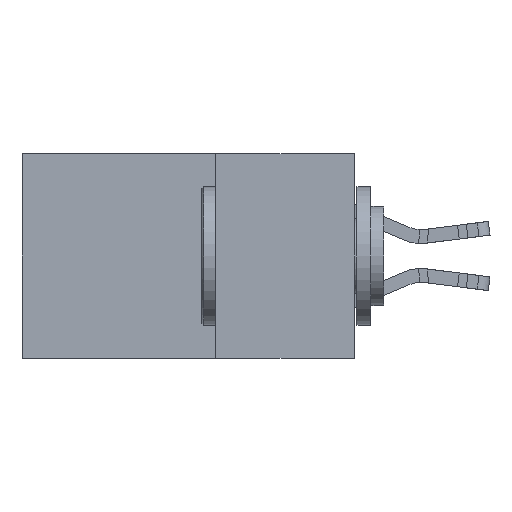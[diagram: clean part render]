
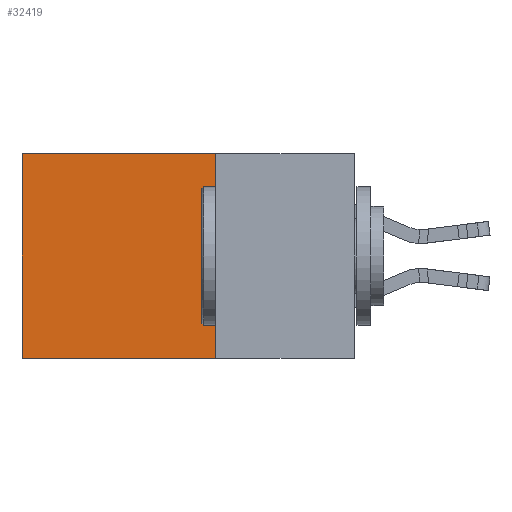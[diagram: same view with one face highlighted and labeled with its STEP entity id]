
A CAD part, left-side view. The second image highlights one B-rep face of the part: STEP entity #32419.
In plain terms, the highlighted planar face has unit normal (-1, 0, 0).
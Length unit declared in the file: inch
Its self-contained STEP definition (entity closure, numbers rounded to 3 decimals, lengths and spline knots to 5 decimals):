
#545 = EDGE_CURVE ( 'NONE', #3159, #31129, #23903, .T. ) ;
#954 = AXIS2_PLACEMENT_3D ( 'NONE', #7554, #33382, #17933 ) ;
#1598 = VECTOR ( 'NONE', #5966, 39.37008 ) ;
#2440 = DIRECTION ( 'NONE',  ( 0., 0., -1. ) ) ;
#2463 = CARTESIAN_POINT ( 'NONE',  ( 0.298, 0.25, -0.37 ) ) ;
#3159 = VERTEX_POINT ( 'NONE', #21073 ) ;
#3337 = DIRECTION ( 'NONE',  ( 0., 0., -1. ) ) ;
#4181 = ORIENTED_EDGE ( 'NONE', *, *, #545, .T. ) ;
#4234 = CARTESIAN_POINT ( 'NONE',  ( 0.298, 0.6, -0.37 ) ) ;
#5095 = CARTESIAN_POINT ( 'NONE',  ( 0.298, 0.25, 0. ) ) ;
#5665 = VECTOR ( 'NONE', #2440, 39.37008 ) ;
#5966 = DIRECTION ( 'NONE',  ( 0., 1., 0. ) ) ;
#6204 = VECTOR ( 'NONE', #23265, 39.37008 ) ;
#6705 = ORIENTED_EDGE ( 'NONE', *, *, #30781, .T. ) ;
#7028 = LINE ( 'NONE', #25914, #6204 ) ;
#7332 = VERTEX_POINT ( 'NONE', #2463 ) ;
#7554 = CARTESIAN_POINT ( 'NONE',  ( 0.298, 0.25, 0. ) ) ;
#10186 = FACE_OUTER_BOUND ( 'NONE', #26141, .T. ) ;
#13841 = EDGE_CURVE ( 'NONE', #7332, #22629, #7028, .T. ) ;
#16269 = CARTESIAN_POINT ( 'NONE',  ( 0.298, 0.6, 0. ) ) ;
#17933 = DIRECTION ( 'NONE',  ( 0., 0., -1. ) ) ;
#18131 = ORIENTED_EDGE ( 'NONE', *, *, #27316, .F. ) ;
#19428 = LINE ( 'NONE', #23175, #5665 ) ;
#20895 = ORIENTED_EDGE ( 'NONE', *, *, #13841, .F. ) ;
#21073 = CARTESIAN_POINT ( 'NONE',  ( 0.298, 0.25, 0. ) ) ;
#22629 = VERTEX_POINT ( 'NONE', #4234 ) ;
#23175 = CARTESIAN_POINT ( 'NONE',  ( 0.298, 0.25, 0. ) ) ;
#23265 = DIRECTION ( 'NONE',  ( 0., 1., 0. ) ) ;
#23903 = LINE ( 'NONE', #5095, #1598 ) ;
#25914 = CARTESIAN_POINT ( 'NONE',  ( 0.298, 0.25, -0.37 ) ) ;
#26141 = EDGE_LOOP ( 'NONE', ( #6705, #20895, #18131, #4181 ) ) ;
#27316 = EDGE_CURVE ( 'NONE', #3159, #7332, #19428, .T. ) ;
#27726 = LINE ( 'NONE', #16269, #32903 ) ;
#30589 = CARTESIAN_POINT ( 'NONE',  ( 0.298, 0.6, 0. ) ) ;
#30781 = EDGE_CURVE ( 'NONE', #31129, #22629, #27726, .T. ) ;
#30803 = PLANE ( 'NONE',  #954 ) ;
#31129 = VERTEX_POINT ( 'NONE', #30589 ) ;
#32419 = ADVANCED_FACE ( 'NONE', ( #10186 ), #30803, .F. ) ;
#32903 = VECTOR ( 'NONE', #3337, 39.37008 ) ;
#33382 = DIRECTION ( 'NONE',  ( 1., 0., 0. ) ) ;
